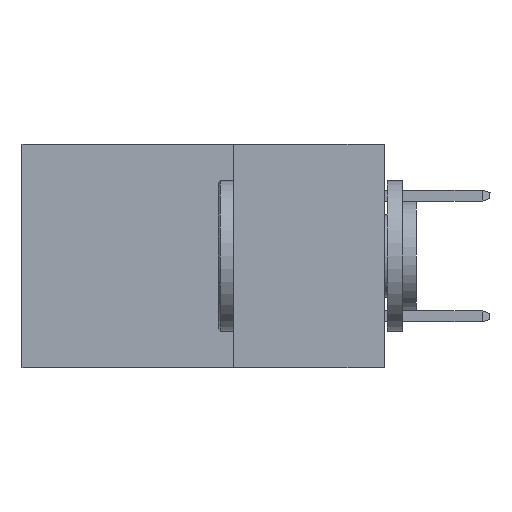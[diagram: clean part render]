
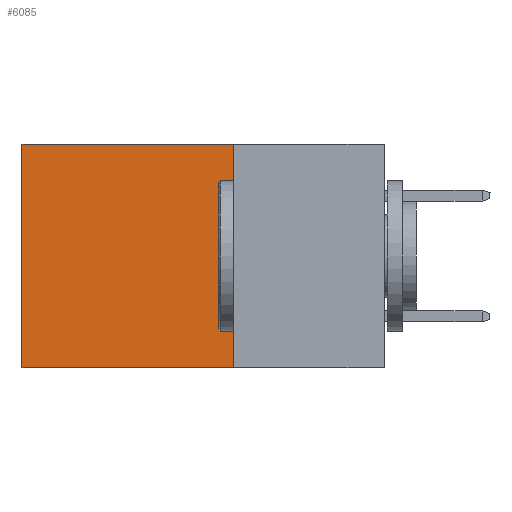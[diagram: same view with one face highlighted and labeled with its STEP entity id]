
A CAD part, left-side view. The second image highlights one B-rep face of the part: STEP entity #6085.
In plain terms, the highlighted planar face has unit normal (-1, 0, 0).
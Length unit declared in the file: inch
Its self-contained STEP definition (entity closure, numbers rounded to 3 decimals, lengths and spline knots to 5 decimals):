
#132 = CARTESIAN_POINT ( 'NONE',  ( 0.298, 0.6, 0. ) ) ;
#554 = CARTESIAN_POINT ( 'NONE',  ( 0.298, 0.25, -0.37 ) ) ;
#804 = ORIENTED_EDGE ( 'NONE', *, *, #3666, .F. ) ;
#1423 = DIRECTION ( 'NONE',  ( 0., 0., -1. ) ) ;
#1463 = CARTESIAN_POINT ( 'NONE',  ( 0.298, 0.25, 0. ) ) ;
#1544 = LINE ( 'NONE', #4163, #1806 ) ;
#1806 = VECTOR ( 'NONE', #10658, 39.37008 ) ;
#1858 = CARTESIAN_POINT ( 'NONE',  ( 0.298, 0.25, 0. ) ) ;
#2156 = CARTESIAN_POINT ( 'NONE',  ( 0.298, 0.25, 0. ) ) ;
#2421 = AXIS2_PLACEMENT_3D ( 'NONE', #2156, #7166, #1423 ) ;
#2979 = LINE ( 'NONE', #132, #4650 ) ;
#3378 = ORIENTED_EDGE ( 'NONE', *, *, #8150, .T. ) ;
#3449 = DIRECTION ( 'NONE',  ( 0., 0., -1. ) ) ;
#3666 = EDGE_CURVE ( 'NONE', #9916, #7530, #1544, .T. ) ;
#3899 = PLANE ( 'NONE',  #2421 ) ;
#4163 = CARTESIAN_POINT ( 'NONE',  ( 0.298, 0.25, 0. ) ) ;
#4390 = LINE ( 'NONE', #8329, #7097 ) ;
#4650 = VECTOR ( 'NONE', #3449, 39.37008 ) ;
#4693 = EDGE_LOOP ( 'NONE', ( #10415, #7899, #804, #3378 ) ) ;
#5723 = VECTOR ( 'NONE', #8829, 39.37008 ) ;
#5883 = FACE_OUTER_BOUND ( 'NONE', #4693, .T. ) ;
#5954 = VERTEX_POINT ( 'NONE', #8295 ) ;
#6085 = ADVANCED_FACE ( 'NONE', ( #5883 ), #3899, .F. ) ;
#7097 = VECTOR ( 'NONE', #8437, 39.37008 ) ;
#7166 = DIRECTION ( 'NONE',  ( 1., 0., 0. ) ) ;
#7315 = VERTEX_POINT ( 'NONE', #7520 ) ;
#7520 = CARTESIAN_POINT ( 'NONE',  ( 0.298, 0.6, 0. ) ) ;
#7530 = VERTEX_POINT ( 'NONE', #554 ) ;
#7899 = ORIENTED_EDGE ( 'NONE', *, *, #8939, .F. ) ;
#8150 = EDGE_CURVE ( 'NONE', #9916, #7315, #10491, .T. ) ;
#8295 = CARTESIAN_POINT ( 'NONE',  ( 0.298, 0.6, -0.37 ) ) ;
#8329 = CARTESIAN_POINT ( 'NONE',  ( 0.298, 0.25, -0.37 ) ) ;
#8437 = DIRECTION ( 'NONE',  ( 0., 1., 0. ) ) ;
#8829 = DIRECTION ( 'NONE',  ( 0., 1., 0. ) ) ;
#8939 = EDGE_CURVE ( 'NONE', #7530, #5954, #4390, .T. ) ;
#9824 = EDGE_CURVE ( 'NONE', #7315, #5954, #2979, .T. ) ;
#9916 = VERTEX_POINT ( 'NONE', #1858 ) ;
#10415 = ORIENTED_EDGE ( 'NONE', *, *, #9824, .T. ) ;
#10491 = LINE ( 'NONE', #1463, #5723 ) ;
#10658 = DIRECTION ( 'NONE',  ( 0., 0., -1. ) ) ;
